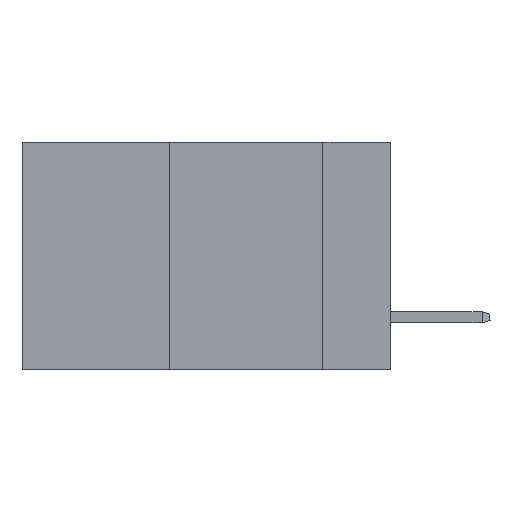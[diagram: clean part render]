
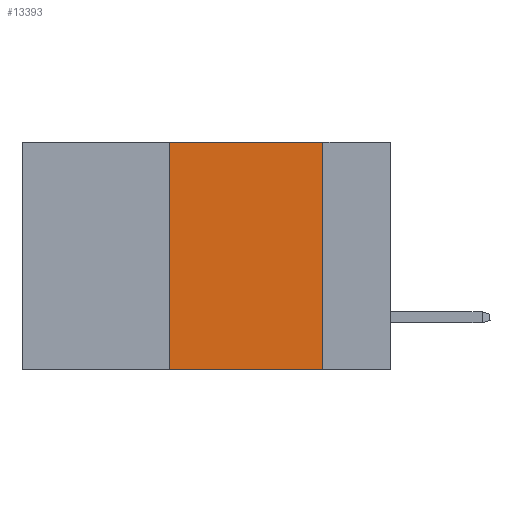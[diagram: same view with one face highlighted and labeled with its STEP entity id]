
A CAD part, left-side view. The second image highlights one B-rep face of the part: STEP entity #13393.
In plain terms, the highlighted planar face has unit normal (-1, 0, 0).
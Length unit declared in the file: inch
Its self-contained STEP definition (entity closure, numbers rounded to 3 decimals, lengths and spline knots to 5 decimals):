
#733 = ORIENTED_EDGE ( 'NONE', *, *, #12735, .T. ) ;
#1122 = CARTESIAN_POINT ( 'NONE',  ( 0., 0.11, 0. ) ) ;
#1206 = ORIENTED_EDGE ( 'NONE', *, *, #4653, .F. ) ;
#1233 = VECTOR ( 'NONE', #25868, 39.37008 ) ;
#1473 = ORIENTED_EDGE ( 'NONE', *, *, #4818, .F. ) ;
#1726 = LINE ( 'NONE', #14204, #21550 ) ;
#2310 = EDGE_CURVE ( 'NONE', #16686, #20158, #21706, .T. ) ;
#4125 = CARTESIAN_POINT ( 'NONE',  ( 0., 0.6, 0. ) ) ;
#4573 = DIRECTION ( 'NONE',  ( 0., -1., 0. ) ) ;
#4653 = EDGE_CURVE ( 'NONE', #7708, #11695, #1726, .T. ) ;
#4818 = EDGE_CURVE ( 'NONE', #11695, #16686, #17618, .T. ) ;
#6201 = DIRECTION ( 'NONE',  ( 0., -1., 0. ) ) ;
#7708 = VERTEX_POINT ( 'NONE', #25501 ) ;
#10167 = CARTESIAN_POINT ( 'NONE',  ( 0., 0.6, 0. ) ) ;
#10429 = DIRECTION ( 'NONE',  ( 1., 0., 0. ) ) ;
#10757 = CARTESIAN_POINT ( 'NONE',  ( 0., 0.6, -0.37 ) ) ;
#11695 = VERTEX_POINT ( 'NONE', #25322 ) ;
#12735 = EDGE_CURVE ( 'NONE', #7708, #20158, #19727, .T. ) ;
#13393 = ADVANCED_FACE ( 'NONE', ( #17722 ), #13885, .F. ) ;
#13885 = PLANE ( 'NONE',  #18548 ) ;
#14204 = CARTESIAN_POINT ( 'NONE',  ( 0., 0.36, 0. ) ) ;
#14719 = VECTOR ( 'NONE', #6201, 39.37008 ) ;
#16686 = VERTEX_POINT ( 'NONE', #1122 ) ;
#17618 = LINE ( 'NONE', #4125, #14719 ) ;
#17722 = FACE_OUTER_BOUND ( 'NONE', #20484, .T. ) ;
#17961 = ORIENTED_EDGE ( 'NONE', *, *, #2310, .F. ) ;
#18408 = VECTOR ( 'NONE', #4573, 39.37008 ) ;
#18548 = AXIS2_PLACEMENT_3D ( 'NONE', #10167, #10429, #20931 ) ;
#19530 = CARTESIAN_POINT ( 'NONE',  ( 0., 0.11, -0.37 ) ) ;
#19727 = LINE ( 'NONE', #10757, #18408 ) ;
#20158 = VERTEX_POINT ( 'NONE', #19530 ) ;
#20484 = EDGE_LOOP ( 'NONE', ( #17961, #1473, #1206, #733 ) ) ;
#20931 = DIRECTION ( 'NONE',  ( 0., 0., -1. ) ) ;
#21550 = VECTOR ( 'NONE', #22544, 39.37008 ) ;
#21706 = LINE ( 'NONE', #26114, #1233 ) ;
#22544 = DIRECTION ( 'NONE',  ( 0., 0., 1. ) ) ;
#25322 = CARTESIAN_POINT ( 'NONE',  ( 0., 0.36, 0. ) ) ;
#25501 = CARTESIAN_POINT ( 'NONE',  ( 0., 0.36, -0.37 ) ) ;
#25868 = DIRECTION ( 'NONE',  ( 0., 0., -1. ) ) ;
#26114 = CARTESIAN_POINT ( 'NONE',  ( 0., 0.11, 0. ) ) ;
